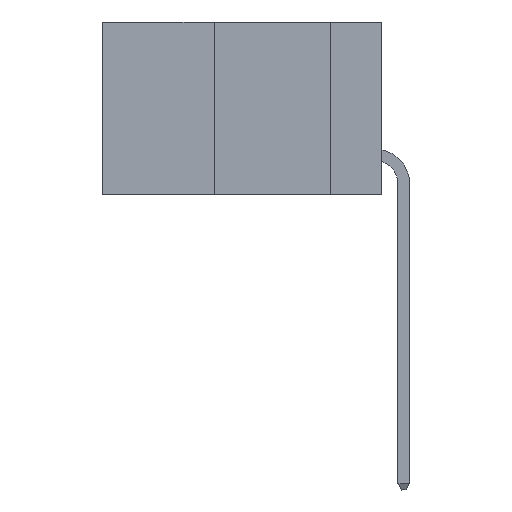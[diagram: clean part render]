
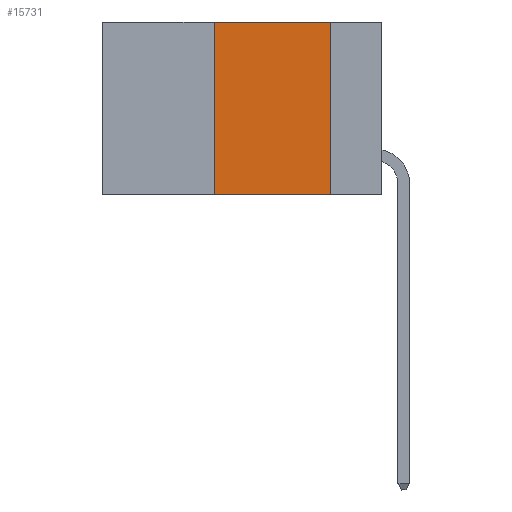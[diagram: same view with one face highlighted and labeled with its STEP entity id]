
A CAD part, left-side view. The second image highlights one B-rep face of the part: STEP entity #15731.
In plain terms, the highlighted planar face has unit normal (-1, 0, 0).
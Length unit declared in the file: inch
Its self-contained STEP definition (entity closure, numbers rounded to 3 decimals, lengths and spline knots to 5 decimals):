
#179 = VERTEX_POINT ( 'NONE', #14067 ) ;
#883 = VECTOR ( 'NONE', #19052, 39.37008 ) ;
#1343 = CARTESIAN_POINT ( 'NONE',  ( 0., 0.6, 0. ) ) ;
#1735 = DIRECTION ( 'NONE',  ( 0., -1., 0. ) ) ;
#2180 = FACE_OUTER_BOUND ( 'NONE', #24138, .T. ) ;
#3300 = EDGE_CURVE ( 'NONE', #19162, #179, #20247, .T. ) ;
#6413 = LINE ( 'NONE', #28328, #30763 ) ;
#7290 = DIRECTION ( 'NONE',  ( 0., 0., -1. ) ) ;
#7361 = CARTESIAN_POINT ( 'NONE',  ( 0., 0.6, 0. ) ) ;
#10000 = PLANE ( 'NONE',  #13013 ) ;
#11216 = ORIENTED_EDGE ( 'NONE', *, *, #12165, .F. ) ;
#11244 = CARTESIAN_POINT ( 'NONE',  ( 0., 0.36, -0.37 ) ) ;
#11781 = CARTESIAN_POINT ( 'NONE',  ( 0., 0.11, -0.37 ) ) ;
#11935 = EDGE_CURVE ( 'NONE', #179, #35062, #32557, .T. ) ;
#12165 = EDGE_CURVE ( 'NONE', #18250, #19162, #6413, .T. ) ;
#12255 = LINE ( 'NONE', #18866, #13639 ) ;
#12927 = ORIENTED_EDGE ( 'NONE', *, *, #11935, .F. ) ;
#13013 = AXIS2_PLACEMENT_3D ( 'NONE', #1343, #13043, #7290 ) ;
#13043 = DIRECTION ( 'NONE',  ( 1., 0., 0. ) ) ;
#13639 = VECTOR ( 'NONE', #1735, 39.37008 ) ;
#14067 = CARTESIAN_POINT ( 'NONE',  ( 0., 0.11, 0. ) ) ;
#14717 = CARTESIAN_POINT ( 'NONE',  ( 0., 0.36, 0. ) ) ;
#15731 = ADVANCED_FACE ( 'NONE', ( #2180 ), #10000, .F. ) ;
#17619 = ORIENTED_EDGE ( 'NONE', *, *, #19262, .T. ) ;
#18250 = VERTEX_POINT ( 'NONE', #11244 ) ;
#18866 = CARTESIAN_POINT ( 'NONE',  ( 0., 0.6, -0.37 ) ) ;
#19052 = DIRECTION ( 'NONE',  ( 0., -1., 0. ) ) ;
#19162 = VERTEX_POINT ( 'NONE', #14717 ) ;
#19262 = EDGE_CURVE ( 'NONE', #18250, #35062, #12255, .T. ) ;
#20247 = LINE ( 'NONE', #7361, #883 ) ;
#20816 = VECTOR ( 'NONE', #31507, 39.37008 ) ;
#24138 = EDGE_LOOP ( 'NONE', ( #12927, #34322, #11216, #17619 ) ) ;
#28328 = CARTESIAN_POINT ( 'NONE',  ( 0., 0.36, 0. ) ) ;
#30763 = VECTOR ( 'NONE', #34863, 39.37008 ) ;
#31134 = CARTESIAN_POINT ( 'NONE',  ( 0., 0.11, 0. ) ) ;
#31507 = DIRECTION ( 'NONE',  ( 0., 0., -1. ) ) ;
#32557 = LINE ( 'NONE', #31134, #20816 ) ;
#34322 = ORIENTED_EDGE ( 'NONE', *, *, #3300, .F. ) ;
#34863 = DIRECTION ( 'NONE',  ( 0., 0., 1. ) ) ;
#35062 = VERTEX_POINT ( 'NONE', #11781 ) ;
